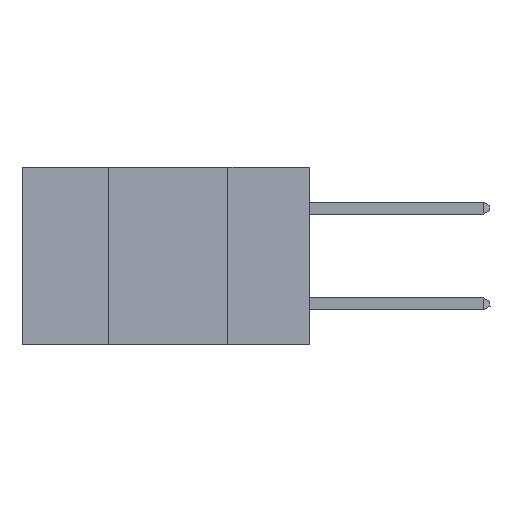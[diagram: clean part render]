
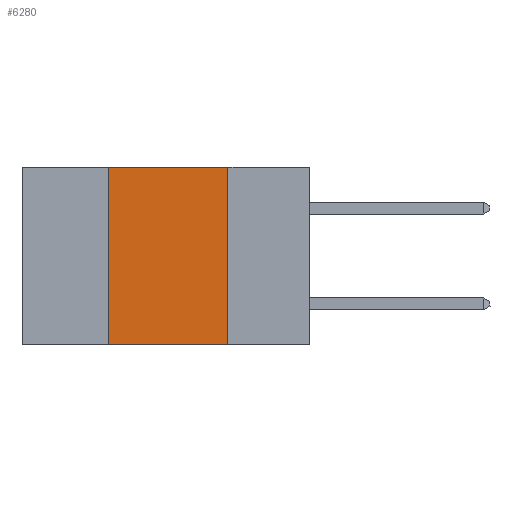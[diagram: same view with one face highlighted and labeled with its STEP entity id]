
A CAD part, left-side view. The second image highlights one B-rep face of the part: STEP entity #6280.
In plain terms, the highlighted planar face has unit normal (-1, 0, 0).
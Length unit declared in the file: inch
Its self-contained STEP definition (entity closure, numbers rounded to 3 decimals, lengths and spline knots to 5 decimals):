
#182 = FACE_OUTER_BOUND ( 'NONE', #16682, .T. ) ;
#632 = LINE ( 'NONE', #19196, #4903 ) ;
#660 = PLANE ( 'NONE',  #8013 ) ;
#1226 = VERTEX_POINT ( 'NONE', #6196 ) ;
#1449 = EDGE_CURVE ( 'NONE', #1839, #9847, #632, .T. ) ;
#1839 = VERTEX_POINT ( 'NONE', #17568 ) ;
#2303 = VECTOR ( 'NONE', #14793, 39.37008 ) ;
#2941 = DIRECTION ( 'NONE',  ( 0., -1., 0. ) ) ;
#3934 = CARTESIAN_POINT ( 'NONE',  ( 0., 0.6, 0. ) ) ;
#4865 = CARTESIAN_POINT ( 'NONE',  ( 0., 0.17, 0. ) ) ;
#4903 = VECTOR ( 'NONE', #12736, 39.37008 ) ;
#5566 = CARTESIAN_POINT ( 'NONE',  ( 0., 0.17, -0.37 ) ) ;
#5704 = EDGE_CURVE ( 'NONE', #9847, #19057, #10424, .T. ) ;
#6196 = CARTESIAN_POINT ( 'NONE',  ( 0., 0.42, -0.37 ) ) ;
#6280 = ADVANCED_FACE ( 'NONE', ( #182 ), #660, .F. ) ;
#8013 = AXIS2_PLACEMENT_3D ( 'NONE', #3934, #17289, #8490 ) ;
#8490 = DIRECTION ( 'NONE',  ( 0., 0., -1. ) ) ;
#8840 = ORIENTED_EDGE ( 'NONE', *, *, #5704, .F. ) ;
#8998 = CARTESIAN_POINT ( 'NONE',  ( 0., 0.6, -0.37 ) ) ;
#9305 = ORIENTED_EDGE ( 'NONE', *, *, #1449, .F. ) ;
#9847 = VERTEX_POINT ( 'NONE', #4865 ) ;
#10424 = LINE ( 'NONE', #19048, #2303 ) ;
#10598 = EDGE_CURVE ( 'NONE', #1226, #1839, #11681, .T. ) ;
#11681 = LINE ( 'NONE', #15604, #16511 ) ;
#11965 = VECTOR ( 'NONE', #2941, 39.37008 ) ;
#12736 = DIRECTION ( 'NONE',  ( 0., -1., 0. ) ) ;
#14793 = DIRECTION ( 'NONE',  ( 0., 0., -1. ) ) ;
#15604 = CARTESIAN_POINT ( 'NONE',  ( 0., 0.42, 0. ) ) ;
#15852 = LINE ( 'NONE', #8998, #11965 ) ;
#16511 = VECTOR ( 'NONE', #17019, 39.37008 ) ;
#16682 = EDGE_LOOP ( 'NONE', ( #8840, #9305, #17085, #17535 ) ) ;
#17019 = DIRECTION ( 'NONE',  ( 0., 0., 1. ) ) ;
#17085 = ORIENTED_EDGE ( 'NONE', *, *, #10598, .F. ) ;
#17289 = DIRECTION ( 'NONE',  ( 1., 0., 0. ) ) ;
#17535 = ORIENTED_EDGE ( 'NONE', *, *, #19318, .T. ) ;
#17568 = CARTESIAN_POINT ( 'NONE',  ( 0., 0.42, 0. ) ) ;
#19048 = CARTESIAN_POINT ( 'NONE',  ( 0., 0.17, 0. ) ) ;
#19057 = VERTEX_POINT ( 'NONE', #5566 ) ;
#19196 = CARTESIAN_POINT ( 'NONE',  ( 0., 0.6, 0. ) ) ;
#19318 = EDGE_CURVE ( 'NONE', #1226, #19057, #15852, .T. ) ;
